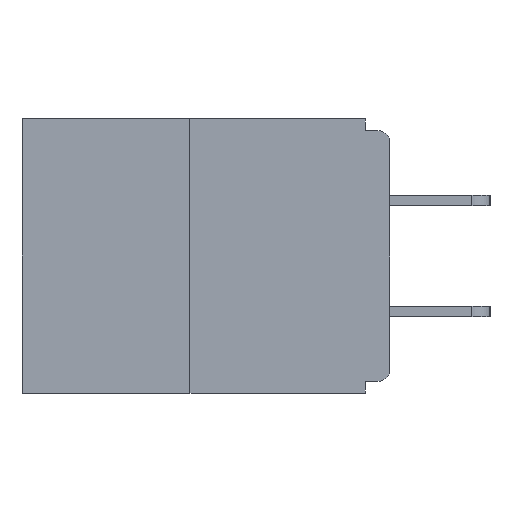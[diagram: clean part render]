
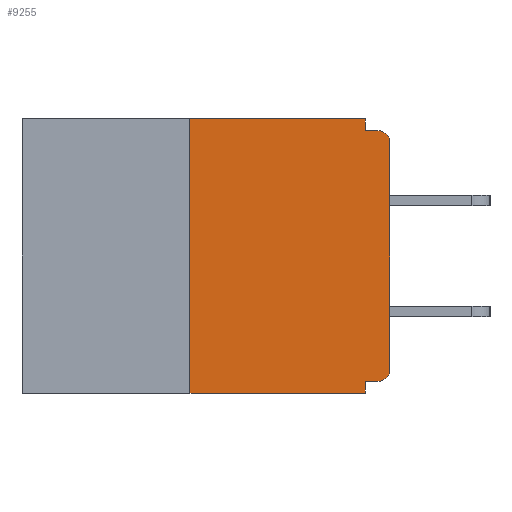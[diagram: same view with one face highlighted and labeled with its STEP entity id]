
A CAD part, left-side view. The second image highlights one B-rep face of the part: STEP entity #9255.
In plain terms, the highlighted planar face has unit normal (-1, 0, 0).
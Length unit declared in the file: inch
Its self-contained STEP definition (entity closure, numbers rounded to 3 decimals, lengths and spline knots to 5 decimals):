
#98 = FACE_OUTER_BOUND ( 'NONE', #12428, .T. ) ;
#424 = CIRCLE ( 'NONE', #14177, 0.015 ) ;
#509 = DIRECTION ( 'NONE',  ( 1., 0., 0. ) ) ;
#593 = VERTEX_POINT ( 'NONE', #8248 ) ;
#770 = EDGE_CURVE ( 'NONE', #15626, #3622, #8172, .T. ) ;
#1350 = ORIENTED_EDGE ( 'NONE', *, *, #22413, .T. ) ;
#1707 = ORIENTED_EDGE ( 'NONE', *, *, #770, .F. ) ;
#1717 = CARTESIAN_POINT ( 'NONE',  ( 0., 0.031, 0. ) ) ;
#1772 = VERTEX_POINT ( 'NONE', #15524 ) ;
#1801 = CARTESIAN_POINT ( 'NONE',  ( 0., 0.015, -0.03 ) ) ;
#2280 = EDGE_CURVE ( 'NONE', #593, #22251, #21122, .T. ) ;
#2731 = ORIENTED_EDGE ( 'NONE', *, *, #4139, .T. ) ;
#2874 = LINE ( 'NONE', #19058, #11351 ) ;
#3456 = VERTEX_POINT ( 'NONE', #11530 ) ;
#3622 = VERTEX_POINT ( 'NONE', #4826 ) ;
#3926 = DIRECTION ( 'NONE',  ( 0., 0., 1. ) ) ;
#3983 = DIRECTION ( 'NONE',  ( 0., 0., 1. ) ) ;
#4050 = ORIENTED_EDGE ( 'NONE', *, *, #4216, .F. ) ;
#4139 = EDGE_CURVE ( 'NONE', #1772, #10890, #20823, .T. ) ;
#4157 = CARTESIAN_POINT ( 'NONE',  ( 0., 0.015, -0.015 ) ) ;
#4216 = EDGE_CURVE ( 'NONE', #3622, #10890, #14674, .T. ) ;
#4575 = LINE ( 'NONE', #21945, #6558 ) ;
#4585 = DIRECTION ( 'NONE',  ( 0., -1., 0. ) ) ;
#4642 = DIRECTION ( 'NONE',  ( 0., -1., 0. ) ) ;
#4826 = CARTESIAN_POINT ( 'NONE',  ( 0., 0.031, -0.328 ) ) ;
#4952 = DIRECTION ( 'NONE',  ( 0., -1., 0. ) ) ;
#5405 = CARTESIAN_POINT ( 'NONE',  ( 0., 0.031, -0.343 ) ) ;
#5828 = VECTOR ( 'NONE', #4952, 39.37008 ) ;
#6114 = VECTOR ( 'NONE', #4642, 39.37008 ) ;
#6453 = VERTEX_POINT ( 'NONE', #17572 ) ;
#6558 = VECTOR ( 'NONE', #3983, 39.37008 ) ;
#6629 = LINE ( 'NONE', #16742, #21612 ) ;
#6854 = ORIENTED_EDGE ( 'NONE', *, *, #15647, .F. ) ;
#7306 = VECTOR ( 'NONE', #14270, 39.37008 ) ;
#7496 = CARTESIAN_POINT ( 'NONE',  ( 0., 0.46, 0. ) ) ;
#7840 = EDGE_CURVE ( 'NONE', #3456, #9177, #424, .T. ) ;
#8155 = EDGE_CURVE ( 'NONE', #15626, #10734, #10915, .T. ) ;
#8172 = LINE ( 'NONE', #21388, #12461 ) ;
#8248 = CARTESIAN_POINT ( 'NONE',  ( 0., 0.25, 0. ) ) ;
#8980 = DIRECTION ( 'NONE',  ( -1., 0., 0. ) ) ;
#9064 = DIRECTION ( 'NONE',  ( 0., 0., -1. ) ) ;
#9177 = VERTEX_POINT ( 'NONE', #4157 ) ;
#9255 = ADVANCED_FACE ( 'NONE', ( #98 ), #22109, .F. ) ;
#9585 = CARTESIAN_POINT ( 'NONE',  ( 0., 0.031, 0. ) ) ;
#10514 = CARTESIAN_POINT ( 'NONE',  ( 0., 0.015, -0.313 ) ) ;
#10602 = CARTESIAN_POINT ( 'NONE',  ( 0., 0.031, -0.343 ) ) ;
#10628 = ORIENTED_EDGE ( 'NONE', *, *, #16935, .F. ) ;
#10734 = VERTEX_POINT ( 'NONE', #20898 ) ;
#10890 = VERTEX_POINT ( 'NONE', #10602 ) ;
#10915 = CIRCLE ( 'NONE', #20223, 0.015 ) ;
#11108 = CARTESIAN_POINT ( 'NONE',  ( 0., 0.015, -0.328 ) ) ;
#11351 = VECTOR ( 'NONE', #4585, 39.37008 ) ;
#11530 = CARTESIAN_POINT ( 'NONE',  ( 0., 0., -0.03 ) ) ;
#12126 = DIRECTION ( 'NONE',  ( -1., 0., 0. ) ) ;
#12428 = EDGE_LOOP ( 'NONE', ( #14596, #6854, #2731, #4050, #1707, #22537, #1350, #18988, #10628, #18020 ) ) ;
#12461 = VECTOR ( 'NONE', #21706, 39.37008 ) ;
#12466 = LINE ( 'NONE', #9585, #18683 ) ;
#13037 = CARTESIAN_POINT ( 'NONE',  ( 0., 0.46, 0. ) ) ;
#14177 = AXIS2_PLACEMENT_3D ( 'NONE', #1801, #8980, #9064 ) ;
#14270 = DIRECTION ( 'NONE',  ( 0., 0., -1. ) ) ;
#14596 = ORIENTED_EDGE ( 'NONE', *, *, #2280, .F. ) ;
#14674 = LINE ( 'NONE', #5405, #7306 ) ;
#15524 = CARTESIAN_POINT ( 'NONE',  ( 0., 0.25, -0.343 ) ) ;
#15626 = VERTEX_POINT ( 'NONE', #11108 ) ;
#15647 = EDGE_CURVE ( 'NONE', #1772, #593, #6629, .T. ) ;
#16002 = DIRECTION ( 'NONE',  ( 0., 0., -1. ) ) ;
#16263 = EDGE_CURVE ( 'NONE', #22251, #6453, #12466, .T. ) ;
#16742 = CARTESIAN_POINT ( 'NONE',  ( 0., 0.25, 0. ) ) ;
#16935 = EDGE_CURVE ( 'NONE', #6453, #9177, #2874, .T. ) ;
#17572 = CARTESIAN_POINT ( 'NONE',  ( 0., 0.031, -0.015 ) ) ;
#18020 = ORIENTED_EDGE ( 'NONE', *, *, #16263, .F. ) ;
#18526 = DIRECTION ( 'NONE',  ( 0., 0., -1. ) ) ;
#18683 = VECTOR ( 'NONE', #18526, 39.37008 ) ;
#18988 = ORIENTED_EDGE ( 'NONE', *, *, #7840, .T. ) ;
#19058 = CARTESIAN_POINT ( 'NONE',  ( 0., 0., -0.015 ) ) ;
#20223 = AXIS2_PLACEMENT_3D ( 'NONE', #10514, #12126, #16002 ) ;
#20823 = LINE ( 'NONE', #21140, #5828 ) ;
#20898 = CARTESIAN_POINT ( 'NONE',  ( 0., 0., -0.313 ) ) ;
#21122 = LINE ( 'NONE', #7496, #6114 ) ;
#21140 = CARTESIAN_POINT ( 'NONE',  ( 0., 0.46, -0.343 ) ) ;
#21388 = CARTESIAN_POINT ( 'NONE',  ( 0., 0., -0.328 ) ) ;
#21612 = VECTOR ( 'NONE', #3926, 39.37008 ) ;
#21706 = DIRECTION ( 'NONE',  ( 0., 1., 0. ) ) ;
#21945 = CARTESIAN_POINT ( 'NONE',  ( 0., 0., 0. ) ) ;
#22037 = DIRECTION ( 'NONE',  ( 0., 0., -1. ) ) ;
#22109 = PLANE ( 'NONE',  #22194 ) ;
#22194 = AXIS2_PLACEMENT_3D ( 'NONE', #13037, #509, #22037 ) ;
#22251 = VERTEX_POINT ( 'NONE', #1717 ) ;
#22413 = EDGE_CURVE ( 'NONE', #10734, #3456, #4575, .T. ) ;
#22537 = ORIENTED_EDGE ( 'NONE', *, *, #8155, .T. ) ;
